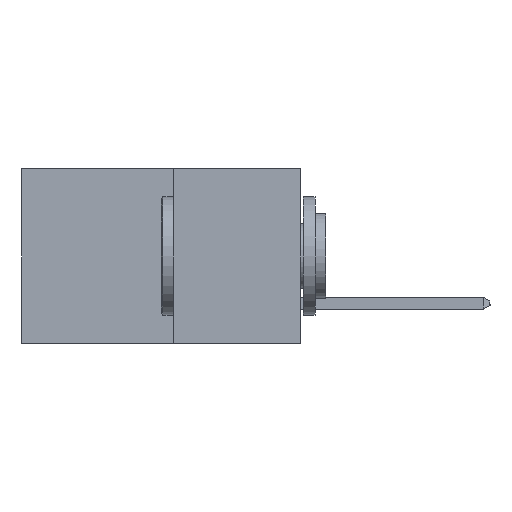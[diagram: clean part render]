
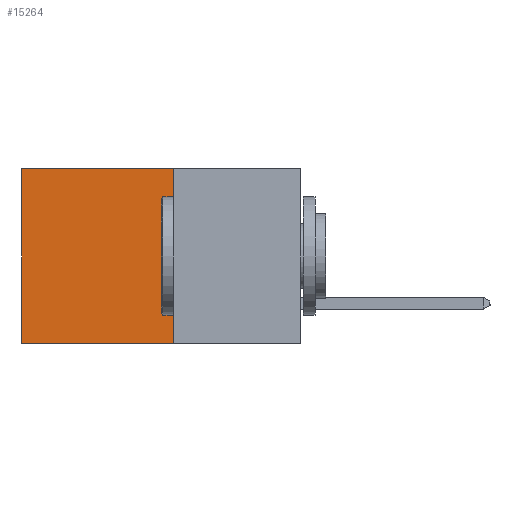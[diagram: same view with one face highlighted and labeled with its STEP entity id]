
A CAD part, left-side view. The second image highlights one B-rep face of the part: STEP entity #15264.
In plain terms, the highlighted planar face has unit normal (-1, 0, 0).
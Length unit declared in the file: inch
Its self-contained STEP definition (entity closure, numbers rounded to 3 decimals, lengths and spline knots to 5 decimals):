
#276 = VECTOR ( 'NONE', #3907, 39.37008 ) ;
#473 = LINE ( 'NONE', #12253, #9897 ) ;
#1740 = EDGE_CURVE ( 'NONE', #3525, #9978, #15337, .T. ) ;
#2276 = ORIENTED_EDGE ( 'NONE', *, *, #1740, .F. ) ;
#2411 = CARTESIAN_POINT ( 'NONE',  ( 0.277, 0.59, -0.37 ) ) ;
#2486 = FACE_OUTER_BOUND ( 'NONE', #6273, .T. ) ;
#2606 = VECTOR ( 'NONE', #12540, 39.37008 ) ;
#2662 = ORIENTED_EDGE ( 'NONE', *, *, #9576, .T. ) ;
#3313 = VERTEX_POINT ( 'NONE', #12964 ) ;
#3525 = VERTEX_POINT ( 'NONE', #9355 ) ;
#3907 = DIRECTION ( 'NONE',  ( 0., 1., 0. ) ) ;
#5042 = CARTESIAN_POINT ( 'NONE',  ( 0.277, 0.59, -0.37 ) ) ;
#5268 = ORIENTED_EDGE ( 'NONE', *, *, #11019, .T. ) ;
#5370 = CARTESIAN_POINT ( 'NONE',  ( 0.277, 0.27, -0.37 ) ) ;
#6102 = DIRECTION ( 'NONE',  ( 0., 1., 0. ) ) ;
#6273 = EDGE_LOOP ( 'NONE', ( #5268, #6385, #2276, #2662 ) ) ;
#6385 = ORIENTED_EDGE ( 'NONE', *, *, #10501, .F. ) ;
#7213 = PLANE ( 'NONE',  #13485 ) ;
#7260 = CARTESIAN_POINT ( 'NONE',  ( 0.277, 0.27, -0.37 ) ) ;
#8070 = LINE ( 'NONE', #2411, #11810 ) ;
#8541 = DIRECTION ( 'NONE',  ( 0., 0., -1. ) ) ;
#9355 = CARTESIAN_POINT ( 'NONE',  ( 0.277, 0.27, 0. ) ) ;
#9576 = EDGE_CURVE ( 'NONE', #3525, #3313, #473, .T. ) ;
#9897 = VECTOR ( 'NONE', #6102, 39.37008 ) ;
#9978 = VERTEX_POINT ( 'NONE', #5370 ) ;
#10489 = VERTEX_POINT ( 'NONE', #5042 ) ;
#10501 = EDGE_CURVE ( 'NONE', #9978, #10489, #12561, .T. ) ;
#10945 = DIRECTION ( 'NONE',  ( 0., 0., -1. ) ) ;
#11019 = EDGE_CURVE ( 'NONE', #3313, #10489, #8070, .T. ) ;
#11234 = CARTESIAN_POINT ( 'NONE',  ( 0.277, 0.27, -0.37 ) ) ;
#11810 = VECTOR ( 'NONE', #10945, 39.37008 ) ;
#12253 = CARTESIAN_POINT ( 'NONE',  ( 0.277, 0.27, 0. ) ) ;
#12540 = DIRECTION ( 'NONE',  ( 0., 0., -1. ) ) ;
#12561 = LINE ( 'NONE', #11234, #276 ) ;
#12964 = CARTESIAN_POINT ( 'NONE',  ( 0.277, 0.59, 0. ) ) ;
#13485 = AXIS2_PLACEMENT_3D ( 'NONE', #7260, #14355, #8541 ) ;
#13698 = CARTESIAN_POINT ( 'NONE',  ( 0.277, 0.27, -0.37 ) ) ;
#14355 = DIRECTION ( 'NONE',  ( 1., 0., 0. ) ) ;
#15264 = ADVANCED_FACE ( 'NONE', ( #2486 ), #7213, .F. ) ;
#15337 = LINE ( 'NONE', #13698, #2606 ) ;
